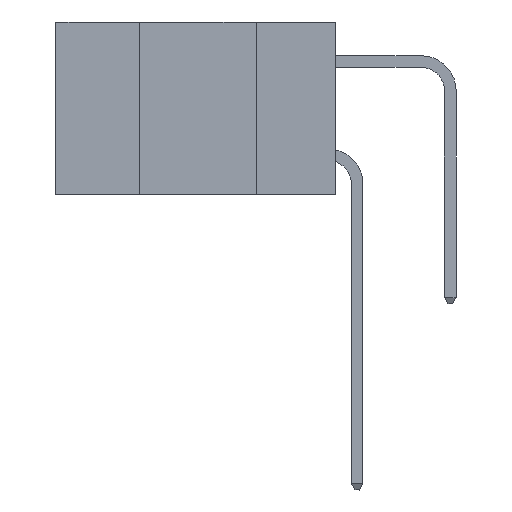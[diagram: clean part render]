
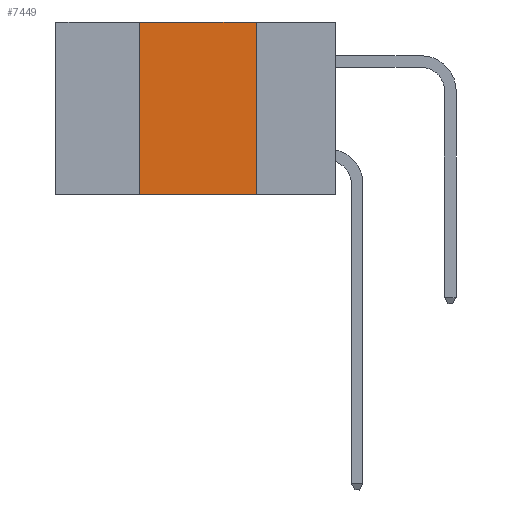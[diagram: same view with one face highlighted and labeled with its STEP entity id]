
A CAD part, left-side view. The second image highlights one B-rep face of the part: STEP entity #7449.
In plain terms, the highlighted planar face has unit normal (-1, 0, 0).
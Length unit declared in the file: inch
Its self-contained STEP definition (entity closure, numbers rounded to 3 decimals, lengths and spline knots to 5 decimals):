
#44 = DIRECTION ( 'NONE',  ( 0., 0., -1. ) ) ;
#871 = VECTOR ( 'NONE', #21363, 39.37008 ) ;
#2543 = EDGE_CURVE ( 'NONE', #12543, #20485, #22049, .T. ) ;
#4151 = CARTESIAN_POINT ( 'NONE',  ( 0., 0.42, 0. ) ) ;
#4174 = LINE ( 'NONE', #19996, #13325 ) ;
#4624 = CARTESIAN_POINT ( 'NONE',  ( 0., 0.17, -0.37 ) ) ;
#5040 = FACE_OUTER_BOUND ( 'NONE', #6621, .T. ) ;
#6528 = EDGE_CURVE ( 'NONE', #16307, #16229, #16044, .T. ) ;
#6621 = EDGE_LOOP ( 'NONE', ( #6925, #19754, #17380, #19573 ) ) ;
#6925 = ORIENTED_EDGE ( 'NONE', *, *, #6528, .F. ) ;
#7211 = CARTESIAN_POINT ( 'NONE',  ( 0., 0.6, 0. ) ) ;
#7449 = ADVANCED_FACE ( 'NONE', ( #5040 ), #17389, .F. ) ;
#7959 = DIRECTION ( 'NONE',  ( 0., -1., 0. ) ) ;
#8025 = CARTESIAN_POINT ( 'NONE',  ( 0., 0.42, 0. ) ) ;
#9582 = CARTESIAN_POINT ( 'NONE',  ( 0., 0.17, 0. ) ) ;
#10670 = EDGE_CURVE ( 'NONE', #12543, #16229, #18991, .T. ) ;
#11305 = DIRECTION ( 'NONE',  ( 0., 0., 1. ) ) ;
#12042 = CARTESIAN_POINT ( 'NONE',  ( 0., 0.6, -0.37 ) ) ;
#12543 = VERTEX_POINT ( 'NONE', #18854 ) ;
#12699 = EDGE_CURVE ( 'NONE', #20485, #16307, #4174, .T. ) ;
#13325 = VECTOR ( 'NONE', #7959, 39.37008 ) ;
#14248 = DIRECTION ( 'NONE',  ( 1., 0., 0. ) ) ;
#14884 = VECTOR ( 'NONE', #11305, 39.37008 ) ;
#16044 = LINE ( 'NONE', #17902, #871 ) ;
#16229 = VERTEX_POINT ( 'NONE', #4624 ) ;
#16307 = VERTEX_POINT ( 'NONE', #9582 ) ;
#17011 = VECTOR ( 'NONE', #20725, 39.37008 ) ;
#17380 = ORIENTED_EDGE ( 'NONE', *, *, #2543, .F. ) ;
#17389 = PLANE ( 'NONE',  #18935 ) ;
#17902 = CARTESIAN_POINT ( 'NONE',  ( 0., 0.17, 0. ) ) ;
#18854 = CARTESIAN_POINT ( 'NONE',  ( 0., 0.42, -0.37 ) ) ;
#18935 = AXIS2_PLACEMENT_3D ( 'NONE', #7211, #14248, #44 ) ;
#18991 = LINE ( 'NONE', #12042, #17011 ) ;
#19573 = ORIENTED_EDGE ( 'NONE', *, *, #10670, .T. ) ;
#19754 = ORIENTED_EDGE ( 'NONE', *, *, #12699, .F. ) ;
#19996 = CARTESIAN_POINT ( 'NONE',  ( 0., 0.6, 0. ) ) ;
#20485 = VERTEX_POINT ( 'NONE', #8025 ) ;
#20725 = DIRECTION ( 'NONE',  ( 0., -1., 0. ) ) ;
#21363 = DIRECTION ( 'NONE',  ( 0., 0., -1. ) ) ;
#22049 = LINE ( 'NONE', #4151, #14884 ) ;
